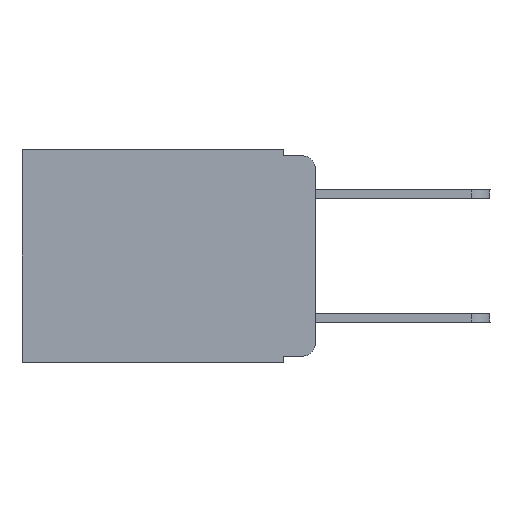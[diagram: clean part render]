
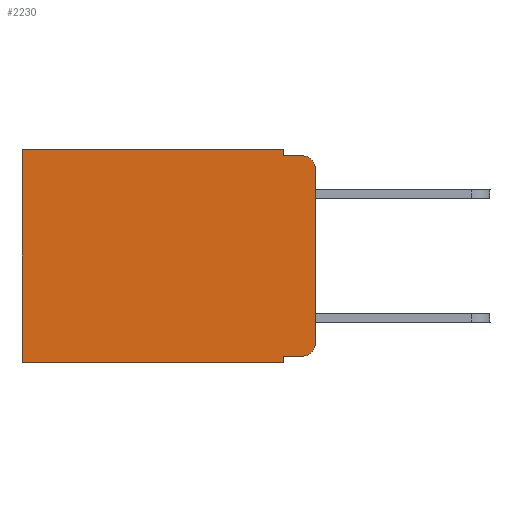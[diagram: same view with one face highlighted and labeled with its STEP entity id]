
A CAD part, left-side view. The second image highlights one B-rep face of the part: STEP entity #2230.
In plain terms, the highlighted planar face has unit normal (-1, 0, 0).
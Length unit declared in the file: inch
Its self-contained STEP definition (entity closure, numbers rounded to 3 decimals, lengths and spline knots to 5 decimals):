
#142 = CARTESIAN_POINT ( 'NONE',  ( 0.298, 0.02, -0.03 ) ) ;
#341 = EDGE_CURVE ( 'NONE', #2690, #12222, #6039, .T. ) ;
#898 = VECTOR ( 'NONE', #2002, 39.37008 ) ;
#962 = VERTEX_POINT ( 'NONE', #2223 ) ;
#1058 = EDGE_CURVE ( 'NONE', #11149, #6593, #11564, .T. ) ;
#1108 = CARTESIAN_POINT ( 'NONE',  ( 0.298, 0.051, 0. ) ) ;
#1346 = DIRECTION ( 'NONE',  ( 0., 0., -1. ) ) ;
#1347 = EDGE_LOOP ( 'NONE', ( #4854, #11065, #12975, #8209, #2590, #5647, #4525, #8437, #5267, #4230 ) ) ;
#1430 = VERTEX_POINT ( 'NONE', #6371 ) ;
#1497 = VECTOR ( 'NONE', #9732, 39.37008 ) ;
#1714 = DIRECTION ( 'NONE',  ( 0., -1., 0. ) ) ;
#1821 = AXIS2_PLACEMENT_3D ( 'NONE', #12329, #10256, #5004 ) ;
#2002 = DIRECTION ( 'NONE',  ( 0., 0., -1. ) ) ;
#2103 = DIRECTION ( 'NONE',  ( 0., 0., -1. ) ) ;
#2142 = VECTOR ( 'NONE', #1346, 39.37008 ) ;
#2210 = CARTESIAN_POINT ( 'NONE',  ( 0.298, 0.02, -0.333 ) ) ;
#2223 = CARTESIAN_POINT ( 'NONE',  ( 0.298, 0.02, -0.01 ) ) ;
#2230 = ADVANCED_FACE ( 'NONE', ( #6133 ), #5066, .F. ) ;
#2590 = ORIENTED_EDGE ( 'NONE', *, *, #9258, .T. ) ;
#2623 = VERTEX_POINT ( 'NONE', #12030 ) ;
#2660 = VERTEX_POINT ( 'NONE', #3147 ) ;
#2690 = VERTEX_POINT ( 'NONE', #2210 ) ;
#3147 = CARTESIAN_POINT ( 'NONE',  ( 0.298, 0.051, -0.343 ) ) ;
#3383 = CARTESIAN_POINT ( 'NONE',  ( 0.298, 0.051, -0.333 ) ) ;
#3519 = LINE ( 'NONE', #9664, #1497 ) ;
#3597 = EDGE_CURVE ( 'NONE', #2623, #962, #6440, .T. ) ;
#3719 = CARTESIAN_POINT ( 'NONE',  ( 0.298, 0.051, -0.01 ) ) ;
#4230 = ORIENTED_EDGE ( 'NONE', *, *, #341, .T. ) ;
#4256 = EDGE_CURVE ( 'NONE', #2623, #12222, #8787, .T. ) ;
#4525 = ORIENTED_EDGE ( 'NONE', *, *, #11150, .F. ) ;
#4854 = ORIENTED_EDGE ( 'NONE', *, *, #4256, .F. ) ;
#4880 = DIRECTION ( 'NONE',  ( -1., 0., 0. ) ) ;
#5004 = DIRECTION ( 'NONE',  ( 0., 0., -1. ) ) ;
#5066 = PLANE ( 'NONE',  #1821 ) ;
#5267 = ORIENTED_EDGE ( 'NONE', *, *, #10821, .T. ) ;
#5287 = VECTOR ( 'NONE', #6629, 39.37008 ) ;
#5556 = VECTOR ( 'NONE', #11325, 39.37008 ) ;
#5647 = ORIENTED_EDGE ( 'NONE', *, *, #1058, .T. ) ;
#5873 = VERTEX_POINT ( 'NONE', #3383 ) ;
#5947 = CARTESIAN_POINT ( 'NONE',  ( 0.298, 0.051, -0.01 ) ) ;
#6039 = CIRCLE ( 'NONE', #12496, 0.02 ) ;
#6133 = FACE_OUTER_BOUND ( 'NONE', #1347, .T. ) ;
#6141 = LINE ( 'NONE', #1108, #5556 ) ;
#6170 = CARTESIAN_POINT ( 'NONE',  ( 0.298, 0., -0.313 ) ) ;
#6297 = CARTESIAN_POINT ( 'NONE',  ( 0.298, 0., 0. ) ) ;
#6371 = CARTESIAN_POINT ( 'NONE',  ( 0.298, 0.051, 0. ) ) ;
#6425 = LINE ( 'NONE', #6297, #11362 ) ;
#6440 = CIRCLE ( 'NONE', #6780, 0.02 ) ;
#6593 = VERTEX_POINT ( 'NONE', #6795 ) ;
#6629 = DIRECTION ( 'NONE',  ( 0., 0., -1. ) ) ;
#6780 = AXIS2_PLACEMENT_3D ( 'NONE', #142, #13281, #2103 ) ;
#6795 = CARTESIAN_POINT ( 'NONE',  ( 0.298, 0.473, -0.343 ) ) ;
#7773 = CARTESIAN_POINT ( 'NONE',  ( 0.298, 0.02, -0.313 ) ) ;
#7818 = DIRECTION ( 'NONE',  ( 0., -1., 0. ) ) ;
#8157 = VECTOR ( 'NONE', #1714, 39.37008 ) ;
#8209 = ORIENTED_EDGE ( 'NONE', *, *, #8354, .F. ) ;
#8354 = EDGE_CURVE ( 'NONE', #1430, #12368, #6141, .T. ) ;
#8437 = ORIENTED_EDGE ( 'NONE', *, *, #13148, .F. ) ;
#8787 = LINE ( 'NONE', #9604, #5287 ) ;
#8791 = LINE ( 'NONE', #10941, #8157 ) ;
#8928 = DIRECTION ( 'NONE',  ( 0., 0., -1. ) ) ;
#9258 = EDGE_CURVE ( 'NONE', #1430, #11149, #6425, .T. ) ;
#9604 = CARTESIAN_POINT ( 'NONE',  ( 0.298, 0., 0. ) ) ;
#9664 = CARTESIAN_POINT ( 'NONE',  ( 0.298, 0., -0.343 ) ) ;
#9732 = DIRECTION ( 'NONE',  ( 0., 1., 0. ) ) ;
#10217 = LINE ( 'NONE', #12290, #898 ) ;
#10256 = DIRECTION ( 'NONE',  ( 1., 0., 0. ) ) ;
#10550 = DIRECTION ( 'NONE',  ( 0., 1., 0. ) ) ;
#10571 = CARTESIAN_POINT ( 'NONE',  ( 0.298, 0.473, 0. ) ) ;
#10821 = EDGE_CURVE ( 'NONE', #5873, #2690, #8791, .T. ) ;
#10941 = CARTESIAN_POINT ( 'NONE',  ( 0.298, 0.051, -0.333 ) ) ;
#11065 = ORIENTED_EDGE ( 'NONE', *, *, #3597, .T. ) ;
#11149 = VERTEX_POINT ( 'NONE', #11666 ) ;
#11150 = EDGE_CURVE ( 'NONE', #2660, #6593, #3519, .T. ) ;
#11325 = DIRECTION ( 'NONE',  ( 0., 0., -1. ) ) ;
#11362 = VECTOR ( 'NONE', #10550, 39.37008 ) ;
#11564 = LINE ( 'NONE', #10571, #2142 ) ;
#11666 = CARTESIAN_POINT ( 'NONE',  ( 0.298, 0.473, 0. ) ) ;
#12030 = CARTESIAN_POINT ( 'NONE',  ( 0.298, 0., -0.03 ) ) ;
#12046 = VECTOR ( 'NONE', #7818, 39.37008 ) ;
#12222 = VERTEX_POINT ( 'NONE', #6170 ) ;
#12290 = CARTESIAN_POINT ( 'NONE',  ( 0.298, 0.051, 0. ) ) ;
#12329 = CARTESIAN_POINT ( 'NONE',  ( 0.298, 0., 0. ) ) ;
#12368 = VERTEX_POINT ( 'NONE', #5947 ) ;
#12496 = AXIS2_PLACEMENT_3D ( 'NONE', #7773, #4880, #8928 ) ;
#12641 = EDGE_CURVE ( 'NONE', #12368, #962, #12820, .T. ) ;
#12820 = LINE ( 'NONE', #3719, #12046 ) ;
#12975 = ORIENTED_EDGE ( 'NONE', *, *, #12641, .F. ) ;
#13148 = EDGE_CURVE ( 'NONE', #5873, #2660, #10217, .T. ) ;
#13281 = DIRECTION ( 'NONE',  ( -1., 0., 0. ) ) ;
